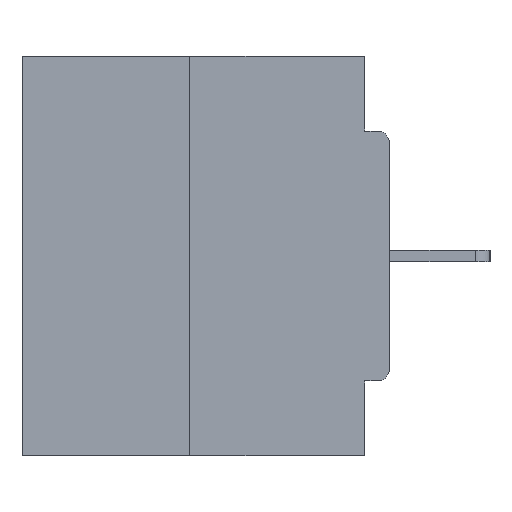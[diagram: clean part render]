
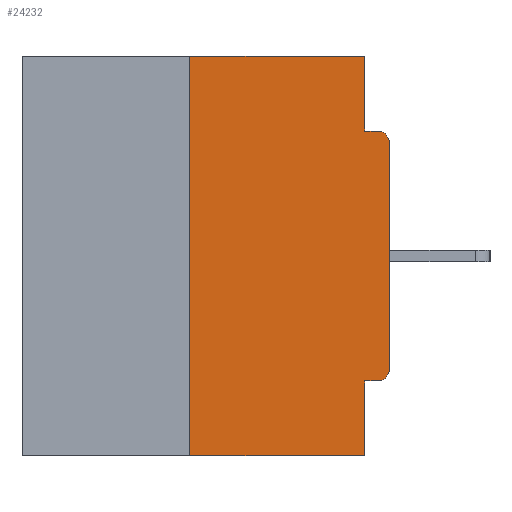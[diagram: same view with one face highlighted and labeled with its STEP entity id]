
A CAD part, left-side view. The second image highlights one B-rep face of the part: STEP entity #24232.
In plain terms, the highlighted planar face has unit normal (-1, 0, 0).
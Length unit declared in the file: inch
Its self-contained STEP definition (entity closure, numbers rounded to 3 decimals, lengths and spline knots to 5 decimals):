
#461 = CARTESIAN_POINT ( 'NONE',  ( 0., 0.031, 0. ) ) ;
#520 = VERTEX_POINT ( 'NONE', #21114 ) ;
#623 = VERTEX_POINT ( 'NONE', #9039 ) ;
#780 = CARTESIAN_POINT ( 'NONE',  ( 0., 0.031, 0. ) ) ;
#846 = DIRECTION ( 'NONE',  ( 0., 0., -1. ) ) ;
#1189 = ORIENTED_EDGE ( 'NONE', *, *, #23089, .T. ) ;
#1374 = EDGE_CURVE ( 'NONE', #2759, #29661, #8744, .T. ) ;
#1442 = VECTOR ( 'NONE', #11780, 39.37008 ) ;
#2388 = ORIENTED_EDGE ( 'NONE', *, *, #16901, .F. ) ;
#2481 = LINE ( 'NONE', #22352, #22862 ) ;
#2566 = VECTOR ( 'NONE', #20762, 39.37008 ) ;
#2759 = VERTEX_POINT ( 'NONE', #12059 ) ;
#3410 = CARTESIAN_POINT ( 'NONE',  ( 0., 0., 0. ) ) ;
#3568 = CARTESIAN_POINT ( 'NONE',  ( 0., 0.031, -0.5 ) ) ;
#3728 = EDGE_CURVE ( 'NONE', #26565, #520, #9605, .T. ) ;
#3892 = LINE ( 'NONE', #3410, #27445 ) ;
#4134 = VECTOR ( 'NONE', #14380, 39.37008 ) ;
#5056 = LINE ( 'NONE', #14462, #16544 ) ;
#5175 = VECTOR ( 'NONE', #23671, 39.37008 ) ;
#5212 = VERTEX_POINT ( 'NONE', #17333 ) ;
#5447 = ORIENTED_EDGE ( 'NONE', *, *, #8694, .T. ) ;
#5877 = ORIENTED_EDGE ( 'NONE', *, *, #9980, .F. ) ;
#6213 = EDGE_CURVE ( 'NONE', #5212, #29661, #15487, .T. ) ;
#6302 = DIRECTION ( 'NONE',  ( 0., 0., 1. ) ) ;
#6616 = VERTEX_POINT ( 'NONE', #6663 ) ;
#6663 = CARTESIAN_POINT ( 'NONE',  ( 0., 0., -0.3915 ) ) ;
#6833 = ORIENTED_EDGE ( 'NONE', *, *, #21797, .F. ) ;
#8075 = DIRECTION ( 'NONE',  ( 0., 0., -1. ) ) ;
#8694 = EDGE_CURVE ( 'NONE', #6616, #27918, #3892, .T. ) ;
#8744 = LINE ( 'NONE', #21121, #5175 ) ;
#9039 = CARTESIAN_POINT ( 'NONE',  ( 0., 0.015, -0.0935 ) ) ;
#9605 = LINE ( 'NONE', #780, #4134 ) ;
#9980 = EDGE_CURVE ( 'NONE', #2759, #30485, #5056, .T. ) ;
#11634 = VECTOR ( 'NONE', #22794, 39.37008 ) ;
#11780 = DIRECTION ( 'NONE',  ( 0., 1., 0. ) ) ;
#12003 = CARTESIAN_POINT ( 'NONE',  ( 0., 0., -0.1085 ) ) ;
#12059 = CARTESIAN_POINT ( 'NONE',  ( 0., 0.25, -0.5 ) ) ;
#12076 = ORIENTED_EDGE ( 'NONE', *, *, #6213, .F. ) ;
#12621 = EDGE_CURVE ( 'NONE', #30485, #26565, #2481, .T. ) ;
#12680 = ORIENTED_EDGE ( 'NONE', *, *, #1374, .T. ) ;
#12696 = AXIS2_PLACEMENT_3D ( 'NONE', #24933, #17302, #8075 ) ;
#12798 = CARTESIAN_POINT ( 'NONE',  ( 0., 0.46, 0. ) ) ;
#13264 = DIRECTION ( 'NONE',  ( -1., 0., 0. ) ) ;
#13573 = DIRECTION ( 'NONE',  ( 0., 0., -1. ) ) ;
#13931 = EDGE_CURVE ( 'NONE', #18607, #6616, #24365, .T. ) ;
#14380 = DIRECTION ( 'NONE',  ( 0., 0., -1. ) ) ;
#14462 = CARTESIAN_POINT ( 'NONE',  ( 0., 0.25, 0. ) ) ;
#14520 = CARTESIAN_POINT ( 'NONE',  ( 0., 0.015, -0.4065 ) ) ;
#15487 = LINE ( 'NONE', #25193, #11634 ) ;
#15846 = CARTESIAN_POINT ( 'NONE',  ( 0., 0., -0.0935 ) ) ;
#16159 = CARTESIAN_POINT ( 'NONE',  ( 0., 0.25, 0. ) ) ;
#16385 = LINE ( 'NONE', #28317, #1442 ) ;
#16544 = VECTOR ( 'NONE', #24156, 39.37008 ) ;
#16901 = EDGE_CURVE ( 'NONE', #520, #623, #25384, .T. ) ;
#17302 = DIRECTION ( 'NONE',  ( -1., 0., 0. ) ) ;
#17333 = CARTESIAN_POINT ( 'NONE',  ( 0., 0.031, -0.4065 ) ) ;
#17420 = PLANE ( 'NONE',  #19361 ) ;
#17901 = ORIENTED_EDGE ( 'NONE', *, *, #13931, .T. ) ;
#18607 = VERTEX_POINT ( 'NONE', #14520 ) ;
#19361 = AXIS2_PLACEMENT_3D ( 'NONE', #12798, #27746, #846 ) ;
#20309 = CIRCLE ( 'NONE', #24375, 0.015 ) ;
#20762 = DIRECTION ( 'NONE',  ( 0., -1., 0. ) ) ;
#21114 = CARTESIAN_POINT ( 'NONE',  ( 0., 0.031, -0.0935 ) ) ;
#21121 = CARTESIAN_POINT ( 'NONE',  ( 0., 0.46, -0.5 ) ) ;
#21797 = EDGE_CURVE ( 'NONE', #18607, #5212, #16385, .T. ) ;
#22352 = CARTESIAN_POINT ( 'NONE',  ( 0., 0.46, 0. ) ) ;
#22794 = DIRECTION ( 'NONE',  ( 0., 0., -1. ) ) ;
#22862 = VECTOR ( 'NONE', #27297, 39.37008 ) ;
#23089 = EDGE_CURVE ( 'NONE', #27918, #623, #20309, .T. ) ;
#23671 = DIRECTION ( 'NONE',  ( 0., -1., 0. ) ) ;
#24156 = DIRECTION ( 'NONE',  ( 0., 0., 1. ) ) ;
#24232 = ADVANCED_FACE ( 'NONE', ( #24871 ), #17420, .F. ) ;
#24365 = CIRCLE ( 'NONE', #12696, 0.015 ) ;
#24375 = AXIS2_PLACEMENT_3D ( 'NONE', #28360, #13264, #13573 ) ;
#24871 = FACE_OUTER_BOUND ( 'NONE', #25594, .T. ) ;
#24933 = CARTESIAN_POINT ( 'NONE',  ( 0., 0.015, -0.3915 ) ) ;
#25193 = CARTESIAN_POINT ( 'NONE',  ( 0., 0.031, -0.5 ) ) ;
#25384 = LINE ( 'NONE', #15846, #2566 ) ;
#25594 = EDGE_LOOP ( 'NONE', ( #25887, #5877, #12680, #12076, #6833, #17901, #5447, #1189, #2388, #26276 ) ) ;
#25887 = ORIENTED_EDGE ( 'NONE', *, *, #12621, .F. ) ;
#26276 = ORIENTED_EDGE ( 'NONE', *, *, #3728, .F. ) ;
#26565 = VERTEX_POINT ( 'NONE', #461 ) ;
#27297 = DIRECTION ( 'NONE',  ( 0., -1., 0. ) ) ;
#27445 = VECTOR ( 'NONE', #6302, 39.37008 ) ;
#27746 = DIRECTION ( 'NONE',  ( 1., 0., 0. ) ) ;
#27918 = VERTEX_POINT ( 'NONE', #12003 ) ;
#28317 = CARTESIAN_POINT ( 'NONE',  ( 0., 0., -0.4065 ) ) ;
#28360 = CARTESIAN_POINT ( 'NONE',  ( 0., 0.015, -0.1085 ) ) ;
#29661 = VERTEX_POINT ( 'NONE', #3568 ) ;
#30485 = VERTEX_POINT ( 'NONE', #16159 ) ;
